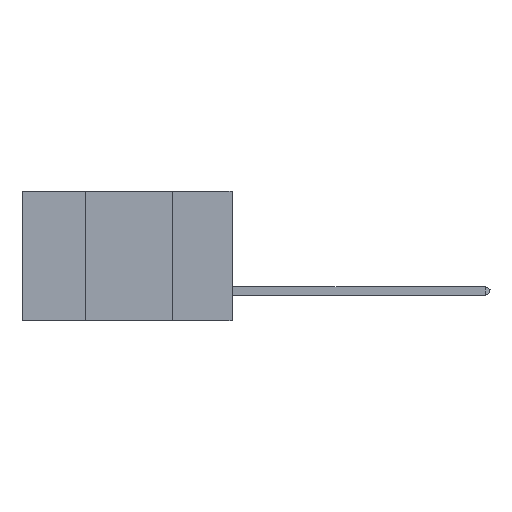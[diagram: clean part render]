
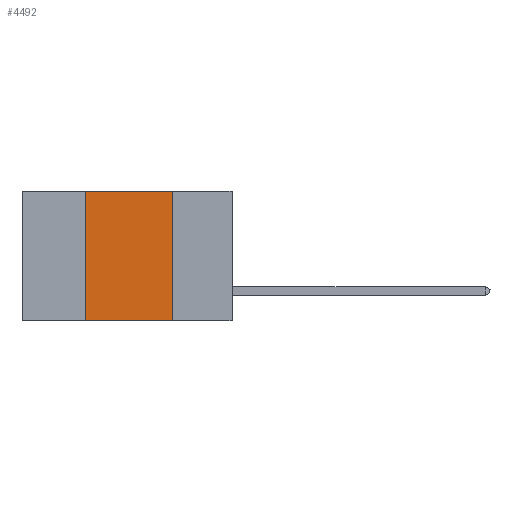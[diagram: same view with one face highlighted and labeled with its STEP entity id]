
A CAD part, left-side view. The second image highlights one B-rep face of the part: STEP entity #4492.
In plain terms, the highlighted planar face has unit normal (-1, 0, 0).
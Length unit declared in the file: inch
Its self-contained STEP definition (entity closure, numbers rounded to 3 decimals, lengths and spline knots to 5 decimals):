
#272 = PLANE ( 'NONE',  #15328 ) ;
#557 = CARTESIAN_POINT ( 'NONE',  ( 0., 0.6, 0. ) ) ;
#718 = EDGE_CURVE ( 'NONE', #20056, #14101, #23235, .T. ) ;
#1909 = DIRECTION ( 'NONE',  ( 0., -1., 0. ) ) ;
#3953 = DIRECTION ( 'NONE',  ( 1., 0., 0. ) ) ;
#4362 = CARTESIAN_POINT ( 'NONE',  ( 0., 0.17, 0. ) ) ;
#4492 = ADVANCED_FACE ( 'NONE', ( #16585 ), #272, .F. ) ;
#5023 = CARTESIAN_POINT ( 'NONE',  ( 0., 0.42, 0. ) ) ;
#7333 = ORIENTED_EDGE ( 'NONE', *, *, #718, .T. ) ;
#8511 = LINE ( 'NONE', #12377, #42927 ) ;
#12377 = CARTESIAN_POINT ( 'NONE',  ( 0., 0.6, 0. ) ) ;
#14007 = VERTEX_POINT ( 'NONE', #29432 ) ;
#14101 = VERTEX_POINT ( 'NONE', #33318 ) ;
#15328 = AXIS2_PLACEMENT_3D ( 'NONE', #557, #3953, #33977 ) ;
#16585 = FACE_OUTER_BOUND ( 'NONE', #24607, .T. ) ;
#17718 = VERTEX_POINT ( 'NONE', #36432 ) ;
#18752 = DIRECTION ( 'NONE',  ( 0., 0., 1. ) ) ;
#19963 = LINE ( 'NONE', #4362, #23128 ) ;
#20056 = VERTEX_POINT ( 'NONE', #26364 ) ;
#23128 = VECTOR ( 'NONE', #38058, 39.37008 ) ;
#23235 = LINE ( 'NONE', #41912, #39386 ) ;
#24607 = EDGE_LOOP ( 'NONE', ( #25781, #34611, #43139, #7333 ) ) ;
#25781 = ORIENTED_EDGE ( 'NONE', *, *, #40557, .F. ) ;
#26364 = CARTESIAN_POINT ( 'NONE',  ( 0., 0.42, -0.37 ) ) ;
#29432 = CARTESIAN_POINT ( 'NONE',  ( 0., 0.17, 0. ) ) ;
#30856 = LINE ( 'NONE', #5023, #37597 ) ;
#32065 = DIRECTION ( 'NONE',  ( 0., -1., 0. ) ) ;
#33318 = CARTESIAN_POINT ( 'NONE',  ( 0., 0.17, -0.37 ) ) ;
#33977 = DIRECTION ( 'NONE',  ( 0., 0., -1. ) ) ;
#34611 = ORIENTED_EDGE ( 'NONE', *, *, #41291, .F. ) ;
#36432 = CARTESIAN_POINT ( 'NONE',  ( 0., 0.42, 0. ) ) ;
#37597 = VECTOR ( 'NONE', #18752, 39.37008 ) ;
#38058 = DIRECTION ( 'NONE',  ( 0., 0., -1. ) ) ;
#39262 = EDGE_CURVE ( 'NONE', #20056, #17718, #30856, .T. ) ;
#39386 = VECTOR ( 'NONE', #1909, 39.37008 ) ;
#40557 = EDGE_CURVE ( 'NONE', #14007, #14101, #19963, .T. ) ;
#41291 = EDGE_CURVE ( 'NONE', #17718, #14007, #8511, .T. ) ;
#41912 = CARTESIAN_POINT ( 'NONE',  ( 0., 0.6, -0.37 ) ) ;
#42927 = VECTOR ( 'NONE', #32065, 39.37008 ) ;
#43139 = ORIENTED_EDGE ( 'NONE', *, *, #39262, .F. ) ;
